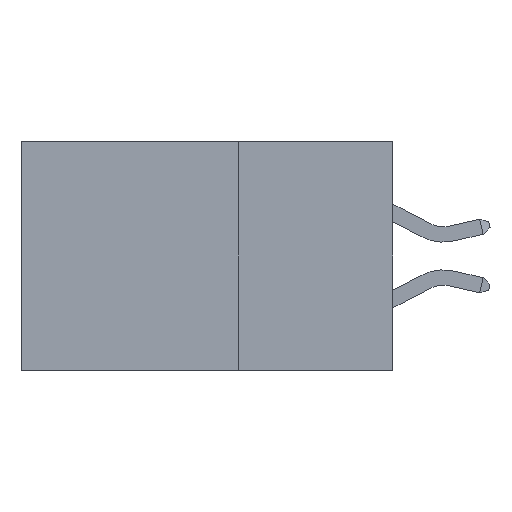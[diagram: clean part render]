
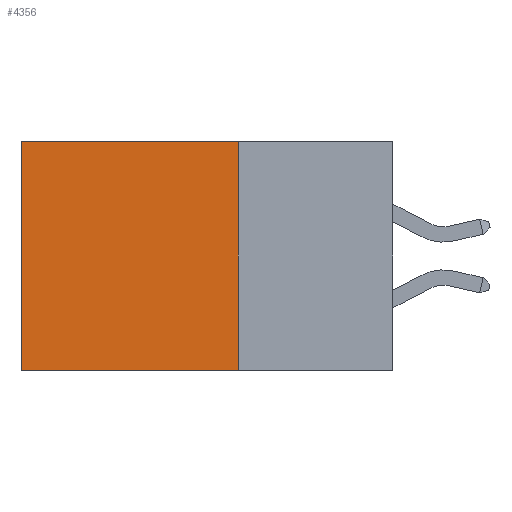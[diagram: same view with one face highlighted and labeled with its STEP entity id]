
A CAD part, left-side view. The second image highlights one B-rep face of the part: STEP entity #4356.
In plain terms, the highlighted planar face has unit normal (-1, 0, 0).
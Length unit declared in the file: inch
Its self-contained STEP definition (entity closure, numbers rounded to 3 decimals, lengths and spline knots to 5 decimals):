
#749 = EDGE_CURVE ( 'NONE', #11619, #4196, #25986, .T. ) ;
#873 = CARTESIAN_POINT ( 'NONE',  ( 0.2875, 0.6, -0.37 ) ) ;
#1005 = AXIS2_PLACEMENT_3D ( 'NONE', #16106, #22147, #7730 ) ;
#1862 = FACE_OUTER_BOUND ( 'NONE', #21177, .T. ) ;
#2171 = VECTOR ( 'NONE', #11230, 39.37008 ) ;
#3103 = CARTESIAN_POINT ( 'NONE',  ( 0.2875, 0.25, -0.37 ) ) ;
#3194 = VECTOR ( 'NONE', #7160, 39.37008 ) ;
#3330 = DIRECTION ( 'NONE',  ( 0., 0., -1. ) ) ;
#3685 = LINE ( 'NONE', #20400, #18833 ) ;
#3729 = ORIENTED_EDGE ( 'NONE', *, *, #23590, .F. ) ;
#4196 = VERTEX_POINT ( 'NONE', #3103 ) ;
#4356 = ADVANCED_FACE ( 'NONE', ( #1862 ), #24339, .F. ) ;
#5579 = DIRECTION ( 'NONE',  ( 0., 1., 0. ) ) ;
#7160 = DIRECTION ( 'NONE',  ( 0., 0., -1. ) ) ;
#7284 = ORIENTED_EDGE ( 'NONE', *, *, #749, .F. ) ;
#7730 = DIRECTION ( 'NONE',  ( 0., 0., -1. ) ) ;
#9460 = ORIENTED_EDGE ( 'NONE', *, *, #10147, .T. ) ;
#10147 = EDGE_CURVE ( 'NONE', #26741, #21289, #15521, .T. ) ;
#11230 = DIRECTION ( 'NONE',  ( 0., 1., 0. ) ) ;
#11619 = VERTEX_POINT ( 'NONE', #14405 ) ;
#11766 = CARTESIAN_POINT ( 'NONE',  ( 0.2875, 0.25, -0.37 ) ) ;
#12767 = CARTESIAN_POINT ( 'NONE',  ( 0.2875, 0.6, 0. ) ) ;
#13817 = LINE ( 'NONE', #11766, #2171 ) ;
#14405 = CARTESIAN_POINT ( 'NONE',  ( 0.2875, 0.25, 0. ) ) ;
#15257 = CARTESIAN_POINT ( 'NONE',  ( 0.2875, 0.25, 0. ) ) ;
#15521 = LINE ( 'NONE', #17987, #25189 ) ;
#16106 = CARTESIAN_POINT ( 'NONE',  ( 0.2875, 0.25, 0. ) ) ;
#17987 = CARTESIAN_POINT ( 'NONE',  ( 0.2875, 0.6, 0. ) ) ;
#18833 = VECTOR ( 'NONE', #5579, 39.37008 ) ;
#20400 = CARTESIAN_POINT ( 'NONE',  ( 0.2875, 0.25, 0. ) ) ;
#21177 = EDGE_LOOP ( 'NONE', ( #9460, #3729, #7284, #22439 ) ) ;
#21289 = VERTEX_POINT ( 'NONE', #873 ) ;
#22147 = DIRECTION ( 'NONE',  ( 1., 0., 0. ) ) ;
#22439 = ORIENTED_EDGE ( 'NONE', *, *, #25573, .T. ) ;
#23590 = EDGE_CURVE ( 'NONE', #4196, #21289, #13817, .T. ) ;
#24339 = PLANE ( 'NONE',  #1005 ) ;
#25189 = VECTOR ( 'NONE', #3330, 39.37008 ) ;
#25573 = EDGE_CURVE ( 'NONE', #11619, #26741, #3685, .T. ) ;
#25986 = LINE ( 'NONE', #15257, #3194 ) ;
#26741 = VERTEX_POINT ( 'NONE', #12767 ) ;
